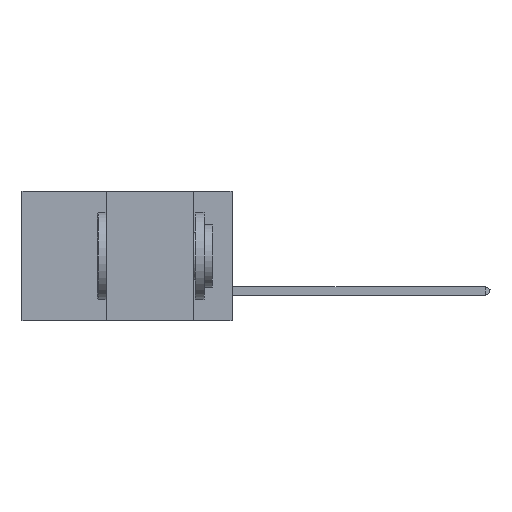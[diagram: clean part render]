
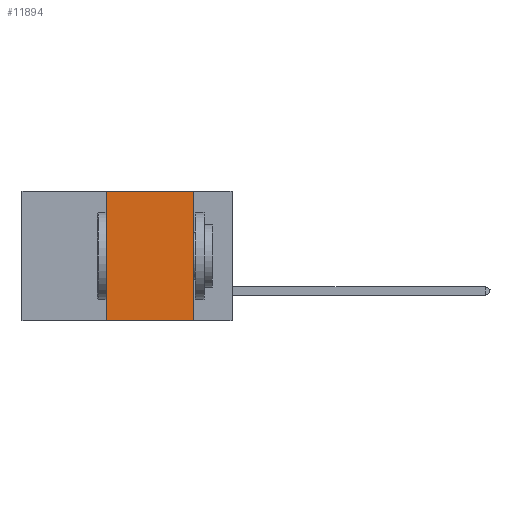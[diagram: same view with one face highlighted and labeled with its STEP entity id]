
A CAD part, left-side view. The second image highlights one B-rep face of the part: STEP entity #11894.
In plain terms, the highlighted planar face has unit normal (-1, 0, 0).
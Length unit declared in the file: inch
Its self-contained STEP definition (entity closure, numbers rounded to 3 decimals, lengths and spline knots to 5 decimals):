
#509 = DIRECTION ( 'NONE',  ( 0., -1., 0. ) ) ;
#656 = DIRECTION ( 'NONE',  ( 0., 0., -1. ) ) ;
#751 = VECTOR ( 'NONE', #14841, 39.37008 ) ;
#1595 = FACE_OUTER_BOUND ( 'NONE', #18634, .T. ) ;
#2515 = VECTOR ( 'NONE', #3704, 39.37008 ) ;
#2526 = EDGE_CURVE ( 'NONE', #8012, #19218, #15066, .T. ) ;
#2717 = VECTOR ( 'NONE', #10075, 39.37008 ) ;
#3402 = EDGE_CURVE ( 'NONE', #18916, #8012, #7648, .T. ) ;
#3485 = AXIS2_PLACEMENT_3D ( 'NONE', #17814, #13027, #656 ) ;
#3569 = CARTESIAN_POINT ( 'NONE',  ( 0., 0.6, -0.37 ) ) ;
#3704 = DIRECTION ( 'NONE',  ( 0., -1., 0. ) ) ;
#4797 = ORIENTED_EDGE ( 'NONE', *, *, #2526, .F. ) ;
#5155 = ORIENTED_EDGE ( 'NONE', *, *, #3402, .F. ) ;
#6653 = ORIENTED_EDGE ( 'NONE', *, *, #9043, .F. ) ;
#7648 = LINE ( 'NONE', #11915, #2717 ) ;
#8012 = VERTEX_POINT ( 'NONE', #11668 ) ;
#9043 = EDGE_CURVE ( 'NONE', #19218, #16409, #12063, .T. ) ;
#9119 = CARTESIAN_POINT ( 'NONE',  ( 0., 0.11, 0. ) ) ;
#9348 = CARTESIAN_POINT ( 'NONE',  ( 0., 0.36, -0.37 ) ) ;
#10075 = DIRECTION ( 'NONE',  ( 0., 0., 1. ) ) ;
#10313 = CARTESIAN_POINT ( 'NONE',  ( 0., 0.11, 0. ) ) ;
#11233 = VECTOR ( 'NONE', #509, 39.37008 ) ;
#11668 = CARTESIAN_POINT ( 'NONE',  ( 0., 0.36, 0. ) ) ;
#11728 = CARTESIAN_POINT ( 'NONE',  ( 0., 0.6, 0. ) ) ;
#11894 = ADVANCED_FACE ( 'NONE', ( #1595 ), #14552, .F. ) ;
#11915 = CARTESIAN_POINT ( 'NONE',  ( 0., 0.36, 0. ) ) ;
#12063 = LINE ( 'NONE', #10313, #751 ) ;
#12918 = LINE ( 'NONE', #3569, #11233 ) ;
#13027 = DIRECTION ( 'NONE',  ( 1., 0., 0. ) ) ;
#14552 = PLANE ( 'NONE',  #3485 ) ;
#14841 = DIRECTION ( 'NONE',  ( 0., 0., -1. ) ) ;
#15066 = LINE ( 'NONE', #11728, #2515 ) ;
#16409 = VERTEX_POINT ( 'NONE', #20485 ) ;
#17814 = CARTESIAN_POINT ( 'NONE',  ( 0., 0.6, 0. ) ) ;
#17844 = EDGE_CURVE ( 'NONE', #18916, #16409, #12918, .T. ) ;
#18634 = EDGE_LOOP ( 'NONE', ( #6653, #4797, #5155, #18793 ) ) ;
#18793 = ORIENTED_EDGE ( 'NONE', *, *, #17844, .T. ) ;
#18916 = VERTEX_POINT ( 'NONE', #9348 ) ;
#19218 = VERTEX_POINT ( 'NONE', #9119 ) ;
#20485 = CARTESIAN_POINT ( 'NONE',  ( 0., 0.11, -0.37 ) ) ;
